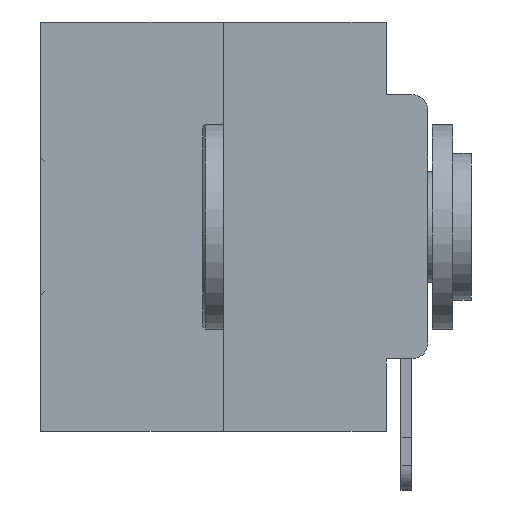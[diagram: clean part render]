
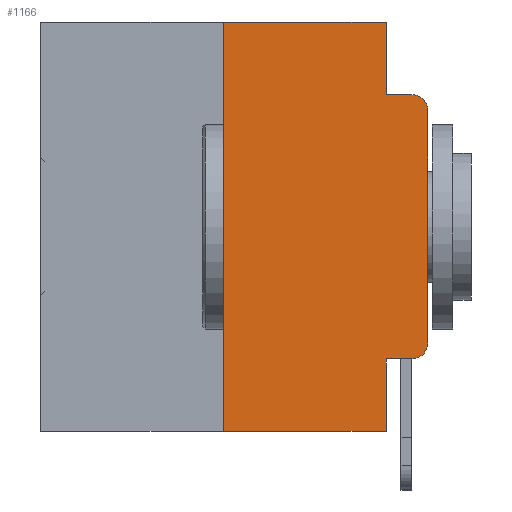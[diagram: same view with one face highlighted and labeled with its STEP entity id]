
A CAD part, left-side view. The second image highlights one B-rep face of the part: STEP entity #1166.
In plain terms, the highlighted planar face has unit normal (-1, 0, 0).
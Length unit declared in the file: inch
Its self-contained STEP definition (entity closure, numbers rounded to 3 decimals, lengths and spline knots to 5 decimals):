
#53 = AXIS2_PLACEMENT_3D ( 'NONE', #4912, #23059, #7636 ) ;
#100 = AXIS2_PLACEMENT_3D ( 'NONE', #17626, #15704, #22128 ) ;
#641 = CARTESIAN_POINT ( 'NONE',  ( 0., 0.25, 0. ) ) ;
#1014 = LINE ( 'NONE', #30515, #7515 ) ;
#1166 = ADVANCED_FACE ( 'NONE', ( #29191 ), #24908, .F. ) ;
#2126 = ORIENTED_EDGE ( 'NONE', *, *, #25822, .F. ) ;
#2204 = VECTOR ( 'NONE', #23191, 39.37008 ) ;
#2346 = ORIENTED_EDGE ( 'NONE', *, *, #22512, .T. ) ;
#2473 = LINE ( 'NONE', #10282, #29146 ) ;
#2657 = ORIENTED_EDGE ( 'NONE', *, *, #29231, .F. ) ;
#2919 = VECTOR ( 'NONE', #30966, 39.37008 ) ;
#3323 = VERTEX_POINT ( 'NONE', #30761 ) ;
#3770 = EDGE_CURVE ( 'NONE', #25907, #10947, #1014, .T. ) ;
#3831 = CARTESIAN_POINT ( 'NONE',  ( 0., 0.051, -0.4115 ) ) ;
#4449 = CIRCLE ( 'NONE', #53, 0.02 ) ;
#4912 = CARTESIAN_POINT ( 'NONE',  ( 0., 0.02, -0.3915 ) ) ;
#5065 = ORIENTED_EDGE ( 'NONE', *, *, #13889, .T. ) ;
#5067 = CARTESIAN_POINT ( 'NONE',  ( 0., 0., 0. ) ) ;
#5188 = DIRECTION ( 'NONE',  ( 0., 0., 1. ) ) ;
#6254 = EDGE_CURVE ( 'NONE', #13728, #7906, #28388, .T. ) ;
#6935 = CARTESIAN_POINT ( 'NONE',  ( 0., 0., -0.1085 ) ) ;
#7483 = CARTESIAN_POINT ( 'NONE',  ( 0., 0.25, 0. ) ) ;
#7515 = VECTOR ( 'NONE', #25504, 39.37008 ) ;
#7521 = CARTESIAN_POINT ( 'NONE',  ( 0., 0.02, -0.1085 ) ) ;
#7636 = DIRECTION ( 'NONE',  ( 0., 0., -1. ) ) ;
#7906 = VERTEX_POINT ( 'NONE', #28078 ) ;
#8522 = VECTOR ( 'NONE', #21662, 39.37008 ) ;
#8730 = VECTOR ( 'NONE', #27863, 39.37008 ) ;
#8936 = LINE ( 'NONE', #30183, #29257 ) ;
#9324 = LINE ( 'NONE', #641, #8522 ) ;
#9972 = VERTEX_POINT ( 'NONE', #14205 ) ;
#10037 = CARTESIAN_POINT ( 'NONE',  ( 0., 0.051, -0.0885 ) ) ;
#10113 = DIRECTION ( 'NONE',  ( 0., 0., -1. ) ) ;
#10207 = LINE ( 'NONE', #28065, #2204 ) ;
#10282 = CARTESIAN_POINT ( 'NONE',  ( 0., 0.051, -0.4115 ) ) ;
#10355 = AXIS2_PLACEMENT_3D ( 'NONE', #7521, #25426, #10113 ) ;
#10947 = VERTEX_POINT ( 'NONE', #25810 ) ;
#11250 = VERTEX_POINT ( 'NONE', #25015 ) ;
#11844 = ORIENTED_EDGE ( 'NONE', *, *, #13239, .T. ) ;
#12985 = DIRECTION ( 'NONE',  ( 0., -1., 0. ) ) ;
#13239 = EDGE_CURVE ( 'NONE', #9972, #13728, #33331, .T. ) ;
#13728 = VERTEX_POINT ( 'NONE', #6935 ) ;
#13889 = EDGE_CURVE ( 'NONE', #11250, #9972, #4449, .T. ) ;
#14205 = CARTESIAN_POINT ( 'NONE',  ( 0., 0., -0.3915 ) ) ;
#14273 = ORIENTED_EDGE ( 'NONE', *, *, #32474, .F. ) ;
#14322 = VERTEX_POINT ( 'NONE', #7483 ) ;
#15704 = DIRECTION ( 'NONE',  ( 1., 0., 0. ) ) ;
#15874 = CARTESIAN_POINT ( 'NONE',  ( 0., 0.051, 0. ) ) ;
#15893 = CARTESIAN_POINT ( 'NONE',  ( 0., 0.25, -0.5 ) ) ;
#17527 = ORIENTED_EDGE ( 'NONE', *, *, #27500, .F. ) ;
#17626 = CARTESIAN_POINT ( 'NONE',  ( 0., 0.473, 0. ) ) ;
#18324 = ORIENTED_EDGE ( 'NONE', *, *, #3770, .T. ) ;
#18664 = VERTEX_POINT ( 'NONE', #28513 ) ;
#19326 = EDGE_LOOP ( 'NONE', ( #11844, #33492, #14273, #29307, #2657, #17527, #18324, #2126, #2346, #5065 ) ) ;
#21662 = DIRECTION ( 'NONE',  ( 0., 0., 1. ) ) ;
#22128 = DIRECTION ( 'NONE',  ( 0., 0., -1. ) ) ;
#22512 = EDGE_CURVE ( 'NONE', #28415, #11250, #2473, .T. ) ;
#23059 = DIRECTION ( 'NONE',  ( -1., 0., 0. ) ) ;
#23191 = DIRECTION ( 'NONE',  ( 0., 0., -1. ) ) ;
#24486 = LINE ( 'NONE', #15874, #2919 ) ;
#24908 = PLANE ( 'NONE',  #100 ) ;
#25015 = CARTESIAN_POINT ( 'NONE',  ( 0., 0.02, -0.4115 ) ) ;
#25426 = DIRECTION ( 'NONE',  ( -1., 0., 0. ) ) ;
#25504 = DIRECTION ( 'NONE',  ( 0., -1., 0. ) ) ;
#25810 = CARTESIAN_POINT ( 'NONE',  ( 0., 0.051, -0.5 ) ) ;
#25822 = EDGE_CURVE ( 'NONE', #28415, #10947, #10207, .T. ) ;
#25907 = VERTEX_POINT ( 'NONE', #15893 ) ;
#26748 = VECTOR ( 'NONE', #5188, 39.37008 ) ;
#27500 = EDGE_CURVE ( 'NONE', #25907, #14322, #9324, .T. ) ;
#27863 = DIRECTION ( 'NONE',  ( 0., -1., 0. ) ) ;
#28065 = CARTESIAN_POINT ( 'NONE',  ( 0., 0.051, 0. ) ) ;
#28078 = CARTESIAN_POINT ( 'NONE',  ( 0., 0.02, -0.0885 ) ) ;
#28271 = LINE ( 'NONE', #10037, #8730 ) ;
#28388 = CIRCLE ( 'NONE', #10355, 0.02 ) ;
#28415 = VERTEX_POINT ( 'NONE', #3831 ) ;
#28513 = CARTESIAN_POINT ( 'NONE',  ( 0., 0.051, 0. ) ) ;
#29146 = VECTOR ( 'NONE', #12985, 39.37008 ) ;
#29191 = FACE_OUTER_BOUND ( 'NONE', #19326, .T. ) ;
#29231 = EDGE_CURVE ( 'NONE', #14322, #18664, #8936, .T. ) ;
#29257 = VECTOR ( 'NONE', #32662, 39.37008 ) ;
#29307 = ORIENTED_EDGE ( 'NONE', *, *, #30836, .F. ) ;
#30183 = CARTESIAN_POINT ( 'NONE',  ( 0., 0.473, 0. ) ) ;
#30515 = CARTESIAN_POINT ( 'NONE',  ( 0., 0.473, -0.5 ) ) ;
#30761 = CARTESIAN_POINT ( 'NONE',  ( 0., 0.051, -0.0885 ) ) ;
#30836 = EDGE_CURVE ( 'NONE', #18664, #3323, #24486, .T. ) ;
#30966 = DIRECTION ( 'NONE',  ( 0., 0., -1. ) ) ;
#32474 = EDGE_CURVE ( 'NONE', #3323, #7906, #28271, .T. ) ;
#32662 = DIRECTION ( 'NONE',  ( 0., -1., 0. ) ) ;
#33331 = LINE ( 'NONE', #5067, #26748 ) ;
#33492 = ORIENTED_EDGE ( 'NONE', *, *, #6254, .T. ) ;
